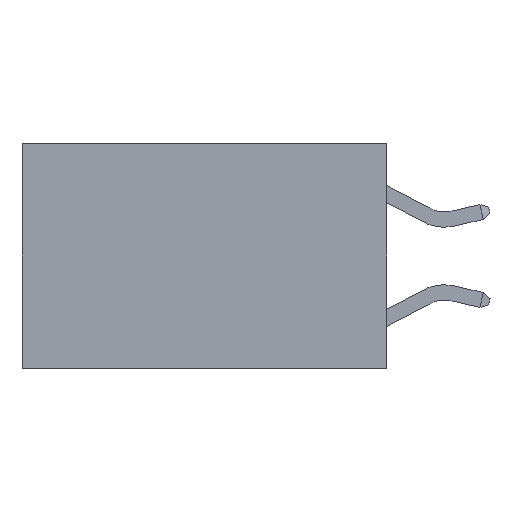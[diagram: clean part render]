
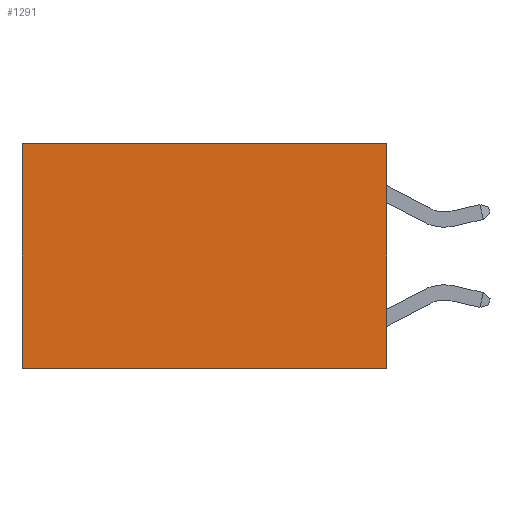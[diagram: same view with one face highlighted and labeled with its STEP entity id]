
A CAD part, left-side view. The second image highlights one B-rep face of the part: STEP entity #1291.
In plain terms, the highlighted planar face has unit normal (-1, 0, 0).
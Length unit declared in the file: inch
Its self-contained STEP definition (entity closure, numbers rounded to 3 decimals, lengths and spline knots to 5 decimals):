
#95 = ORIENTED_EDGE ( 'NONE', *, *, #17723, .F. ) ;
#489 = ORIENTED_EDGE ( 'NONE', *, *, #5912, .T. ) ;
#806 = CARTESIAN_POINT ( 'NONE',  ( 0.2625, 0., 0. ) ) ;
#912 = EDGE_LOOP ( 'NONE', ( #14076, #1526, #95, #489 ) ) ;
#1102 = VECTOR ( 'NONE', #19332, 39.37008 ) ;
#1291 = ADVANCED_FACE ( 'NONE', ( #17617 ), #1448, .F. ) ;
#1448 = PLANE ( 'NONE',  #17717 ) ;
#1526 = ORIENTED_EDGE ( 'NONE', *, *, #14963, .F. ) ;
#1889 = LINE ( 'NONE', #806, #13425 ) ;
#2276 = VECTOR ( 'NONE', #15450, 39.37008 ) ;
#5615 = CARTESIAN_POINT ( 'NONE',  ( 0.2625, 0., -0.37 ) ) ;
#5891 = VECTOR ( 'NONE', #8795, 39.37008 ) ;
#5912 = EDGE_CURVE ( 'NONE', #17385, #19587, #6918, .T. ) ;
#6918 = LINE ( 'NONE', #12339, #2276 ) ;
#7403 = VERTEX_POINT ( 'NONE', #8212 ) ;
#8212 = CARTESIAN_POINT ( 'NONE',  ( 0.2625, 0., -0.37 ) ) ;
#8416 = CARTESIAN_POINT ( 'NONE',  ( 0.2625, 0., 0. ) ) ;
#8795 = DIRECTION ( 'NONE',  ( 0., 1., 0. ) ) ;
#9462 = LINE ( 'NONE', #14745, #1102 ) ;
#10087 = LINE ( 'NONE', #5615, #5891 ) ;
#12339 = CARTESIAN_POINT ( 'NONE',  ( 0.2625, 0., 0. ) ) ;
#13089 = CARTESIAN_POINT ( 'NONE',  ( 0.2625, 0.6, 0. ) ) ;
#13367 = DIRECTION ( 'NONE',  ( 0., 0., -1. ) ) ;
#13425 = VECTOR ( 'NONE', #13367, 39.37008 ) ;
#14076 = ORIENTED_EDGE ( 'NONE', *, *, #18865, .T. ) ;
#14745 = CARTESIAN_POINT ( 'NONE',  ( 0.2625, 0.6, 0. ) ) ;
#14760 = DIRECTION ( 'NONE',  ( 0., 0., -1. ) ) ;
#14963 = EDGE_CURVE ( 'NONE', #7403, #16248, #10087, .T. ) ;
#15450 = DIRECTION ( 'NONE',  ( 0., 1., 0. ) ) ;
#15898 = CARTESIAN_POINT ( 'NONE',  ( 0.2625, 0., 0. ) ) ;
#16248 = VERTEX_POINT ( 'NONE', #19584 ) ;
#17385 = VERTEX_POINT ( 'NONE', #15898 ) ;
#17617 = FACE_OUTER_BOUND ( 'NONE', #912, .T. ) ;
#17717 = AXIS2_PLACEMENT_3D ( 'NONE', #8416, #18786, #14760 ) ;
#17723 = EDGE_CURVE ( 'NONE', #17385, #7403, #1889, .T. ) ;
#18786 = DIRECTION ( 'NONE',  ( 1., 0., 0. ) ) ;
#18865 = EDGE_CURVE ( 'NONE', #19587, #16248, #9462, .T. ) ;
#19332 = DIRECTION ( 'NONE',  ( 0., 0., -1. ) ) ;
#19584 = CARTESIAN_POINT ( 'NONE',  ( 0.2625, 0.6, -0.37 ) ) ;
#19587 = VERTEX_POINT ( 'NONE', #13089 ) ;
